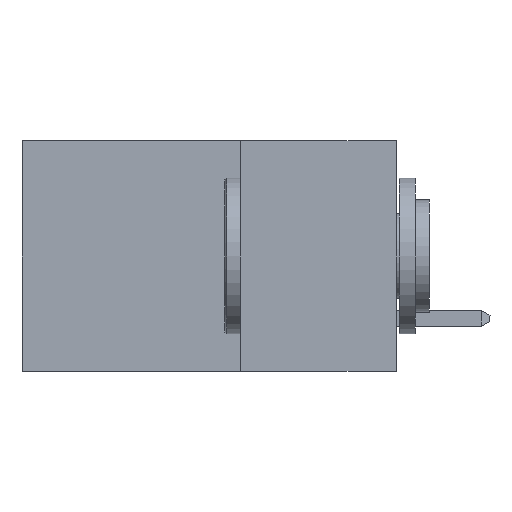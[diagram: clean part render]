
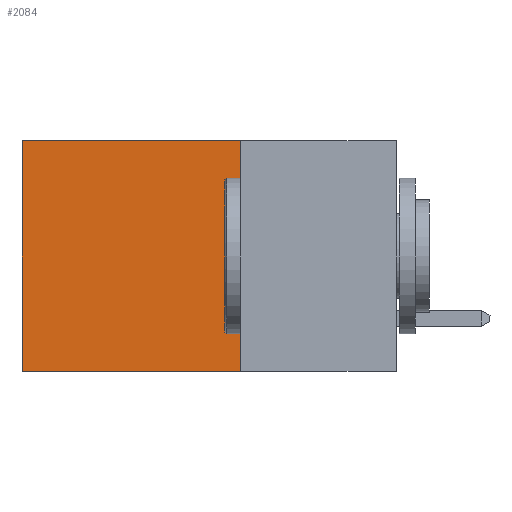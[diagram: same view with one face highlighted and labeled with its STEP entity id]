
A CAD part, left-side view. The second image highlights one B-rep face of the part: STEP entity #2084.
In plain terms, the highlighted planar face has unit normal (-1, 0, 0).
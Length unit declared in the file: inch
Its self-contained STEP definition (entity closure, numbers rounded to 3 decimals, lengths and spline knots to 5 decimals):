
#17 = DIRECTION ( 'NONE',  ( 0., 0., -1. ) ) ;
#129 = LINE ( 'NONE', #1644, #5662 ) ;
#179 = DIRECTION ( 'NONE',  ( 0., 1., 0. ) ) ;
#420 = EDGE_CURVE ( 'NONE', #3212, #741, #129, .T. ) ;
#578 = ORIENTED_EDGE ( 'NONE', *, *, #420, .T. ) ;
#592 = VECTOR ( 'NONE', #179, 39.37008 ) ;
#741 = VERTEX_POINT ( 'NONE', #2740 ) ;
#933 = DIRECTION ( 'NONE',  ( 0., 1., 0. ) ) ;
#979 = LINE ( 'NONE', #5219, #5935 ) ;
#1014 = PLANE ( 'NONE',  #1262 ) ;
#1148 = DIRECTION ( 'NONE',  ( 0., 0., -1. ) ) ;
#1262 = AXIS2_PLACEMENT_3D ( 'NONE', #8652, #7371, #1148 ) ;
#1373 = VERTEX_POINT ( 'NONE', #6308 ) ;
#1644 = CARTESIAN_POINT ( 'NONE',  ( 0.2615, 0.6, -0.37 ) ) ;
#1664 = ORIENTED_EDGE ( 'NONE', *, *, #5133, .T. ) ;
#1699 = CARTESIAN_POINT ( 'NONE',  ( 0.2615, 0.25, 0. ) ) ;
#1715 = EDGE_LOOP ( 'NONE', ( #578, #4421, #8441, #1664 ) ) ;
#2084 = ADVANCED_FACE ( 'NONE', ( #6008 ), #1014, .F. ) ;
#2114 = VERTEX_POINT ( 'NONE', #7277 ) ;
#2717 = CARTESIAN_POINT ( 'NONE',  ( 0.2615, 0.6, 0. ) ) ;
#2740 = CARTESIAN_POINT ( 'NONE',  ( 0.2615, 0.6, -0.37 ) ) ;
#2923 = DIRECTION ( 'NONE',  ( 0., 0., -1. ) ) ;
#3212 = VERTEX_POINT ( 'NONE', #2717 ) ;
#4421 = ORIENTED_EDGE ( 'NONE', *, *, #4748, .F. ) ;
#4573 = EDGE_CURVE ( 'NONE', #2114, #1373, #6341, .T. ) ;
#4748 = EDGE_CURVE ( 'NONE', #1373, #741, #979, .T. ) ;
#5133 = EDGE_CURVE ( 'NONE', #2114, #3212, #5799, .T. ) ;
#5219 = CARTESIAN_POINT ( 'NONE',  ( 0.2615, 0.25, -0.37 ) ) ;
#5660 = VECTOR ( 'NONE', #17, 39.37008 ) ;
#5662 = VECTOR ( 'NONE', #2923, 39.37008 ) ;
#5799 = LINE ( 'NONE', #1699, #592 ) ;
#5935 = VECTOR ( 'NONE', #933, 39.37008 ) ;
#6008 = FACE_OUTER_BOUND ( 'NONE', #1715, .T. ) ;
#6308 = CARTESIAN_POINT ( 'NONE',  ( 0.2615, 0.25, -0.37 ) ) ;
#6341 = LINE ( 'NONE', #6929, #5660 ) ;
#6929 = CARTESIAN_POINT ( 'NONE',  ( 0.2615, 0.25, -0.37 ) ) ;
#7277 = CARTESIAN_POINT ( 'NONE',  ( 0.2615, 0.25, 0. ) ) ;
#7371 = DIRECTION ( 'NONE',  ( 1., 0., 0. ) ) ;
#8441 = ORIENTED_EDGE ( 'NONE', *, *, #4573, .F. ) ;
#8652 = CARTESIAN_POINT ( 'NONE',  ( 0.2615, 0.25, -0.37 ) ) ;
